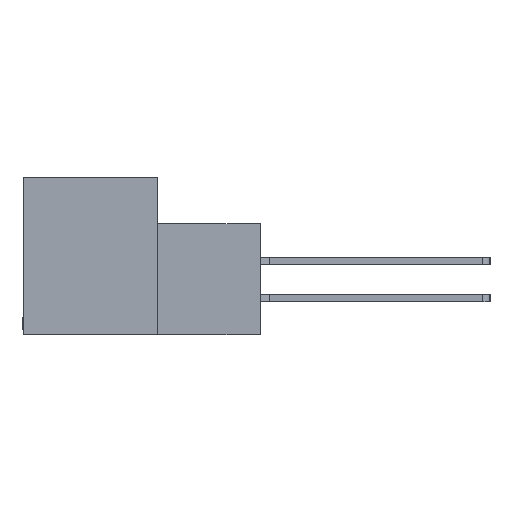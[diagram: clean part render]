
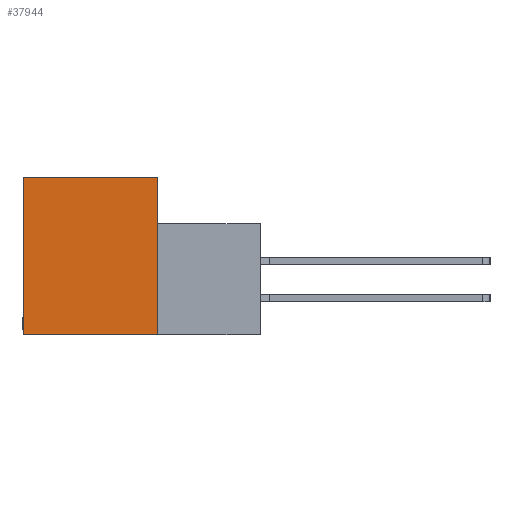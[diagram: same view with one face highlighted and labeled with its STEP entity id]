
A CAD part, left-side view. The second image highlights one B-rep face of the part: STEP entity #37944.
In plain terms, the highlighted planar face has unit normal (-1, 0, 0).
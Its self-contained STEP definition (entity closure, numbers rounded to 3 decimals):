
#742 = CARTESIAN_POINT ( 'NONE',  ( 0., 11.506, -13.487 ) ) ;
#2017 = CARTESIAN_POINT ( 'NONE',  ( 0., 0., -13.487 ) ) ;
#2597 = DIRECTION ( 'NONE',  ( 0., 0., 1. ) ) ;
#3384 = VERTEX_POINT ( 'NONE', #742 ) ;
#3840 = ORIENTED_EDGE ( 'NONE', *, *, #22814, .F. ) ;
#4025 = LINE ( 'NONE', #17672, #14707 ) ;
#4115 = CARTESIAN_POINT ( 'NONE',  ( 0., 0., 0. ) ) ;
#4742 = EDGE_CURVE ( 'NONE', #33960, #3384, #13101, .T. ) ;
#4797 = VECTOR ( 'NONE', #15826, 1000. ) ;
#7147 = LINE ( 'NONE', #15223, #33424 ) ;
#7165 = CARTESIAN_POINT ( 'NONE',  ( 0., 0., 0. ) ) ;
#10103 = FACE_OUTER_BOUND ( 'NONE', #39555, .T. ) ;
#10200 = CARTESIAN_POINT ( 'NONE',  ( 0., 11.506, 0. ) ) ;
#13101 = LINE ( 'NONE', #16801, #27689 ) ;
#13279 = PLANE ( 'NONE',  #15342 ) ;
#13541 = DIRECTION ( 'NONE',  ( 1., 0., 0. ) ) ;
#13616 = VERTEX_POINT ( 'NONE', #10200 ) ;
#13943 = DIRECTION ( 'NONE',  ( 0., 1., 0. ) ) ;
#14707 = VECTOR ( 'NONE', #14829, 1000. ) ;
#14829 = DIRECTION ( 'NONE',  ( 0., 0., -1. ) ) ;
#15223 = CARTESIAN_POINT ( 'NONE',  ( 0., 11.506, -13.487 ) ) ;
#15290 = CARTESIAN_POINT ( 'NONE',  ( 0., 11.506, 0. ) ) ;
#15342 = AXIS2_PLACEMENT_3D ( 'NONE', #7165, #13541, #19803 ) ;
#15826 = DIRECTION ( 'NONE',  ( 0., -1., 0. ) ) ;
#15853 = EDGE_CURVE ( 'NONE', #26813, #33960, #4025, .T. ) ;
#16801 = CARTESIAN_POINT ( 'NONE',  ( 0., -8.814, -13.487 ) ) ;
#17672 = CARTESIAN_POINT ( 'NONE',  ( 0., 0., 0. ) ) ;
#19803 = DIRECTION ( 'NONE',  ( 0., 0., -1. ) ) ;
#21116 = ORIENTED_EDGE ( 'NONE', *, *, #34655, .F. ) ;
#21796 = ORIENTED_EDGE ( 'NONE', *, *, #15853, .F. ) ;
#22814 = EDGE_CURVE ( 'NONE', #3384, #13616, #7147, .T. ) ;
#26813 = VERTEX_POINT ( 'NONE', #4115 ) ;
#27689 = VECTOR ( 'NONE', #13943, 1000. ) ;
#33424 = VECTOR ( 'NONE', #2597, 1000. ) ;
#33960 = VERTEX_POINT ( 'NONE', #2017 ) ;
#34655 = EDGE_CURVE ( 'NONE', #13616, #26813, #37841, .T. ) ;
#37841 = LINE ( 'NONE', #15290, #4797 ) ;
#37944 = ADVANCED_FACE ( 'NONE', ( #10103 ), #13279, .F. ) ;
#38926 = ORIENTED_EDGE ( 'NONE', *, *, #4742, .F. ) ;
#39555 = EDGE_LOOP ( 'NONE', ( #38926, #21796, #21116, #3840 ) ) ;
